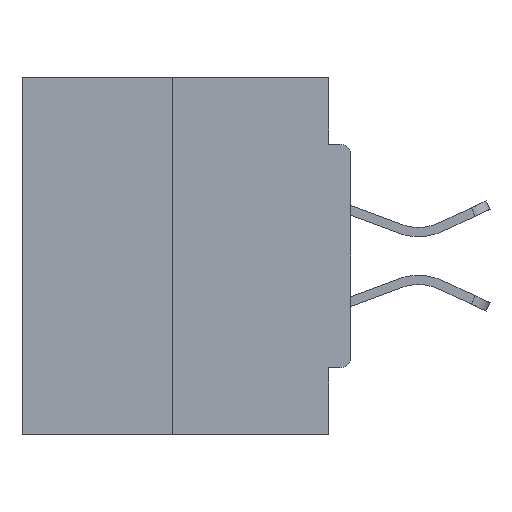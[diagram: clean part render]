
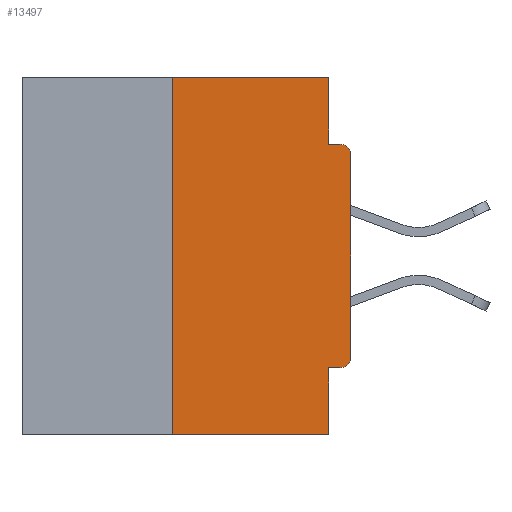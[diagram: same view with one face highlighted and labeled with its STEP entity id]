
A CAD part, left-side view. The second image highlights one B-rep face of the part: STEP entity #13497.
In plain terms, the highlighted planar face has unit normal (-1, 0, 0).
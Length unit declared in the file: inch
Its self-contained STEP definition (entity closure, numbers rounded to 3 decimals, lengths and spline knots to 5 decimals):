
#79 = EDGE_CURVE ( 'NONE', #23908, #3379, #25106, .T. ) ;
#124 = CIRCLE ( 'NONE', #31259, 0.015 ) ;
#161 = CARTESIAN_POINT ( 'NONE',  ( 0., 0.015, -0.1085 ) ) ;
#255 = CARTESIAN_POINT ( 'NONE',  ( 0., 0.031, -0.4065 ) ) ;
#318 = ORIENTED_EDGE ( 'NONE', *, *, #26460, .T. ) ;
#362 = ORIENTED_EDGE ( 'NONE', *, *, #3439, .T. ) ;
#2092 = DIRECTION ( 'NONE',  ( 0., 1., 0. ) ) ;
#2394 = LINE ( 'NONE', #14521, #20376 ) ;
#2426 = ORIENTED_EDGE ( 'NONE', *, *, #20431, .F. ) ;
#2506 = DIRECTION ( 'NONE',  ( 1., 0., 0. ) ) ;
#3024 = LINE ( 'NONE', #3363, #23427 ) ;
#3052 = DIRECTION ( 'NONE',  ( -1., 0., 0. ) ) ;
#3363 = CARTESIAN_POINT ( 'NONE',  ( 0., 0.46, 0. ) ) ;
#3379 = VERTEX_POINT ( 'NONE', #255 ) ;
#3439 = EDGE_CURVE ( 'NONE', #19172, #28922, #10156, .T. ) ;
#3564 = VECTOR ( 'NONE', #4030, 39.37008 ) ;
#4030 = DIRECTION ( 'NONE',  ( 0., -1., 0. ) ) ;
#4635 = EDGE_CURVE ( 'NONE', #23908, #19172, #124, .T. ) ;
#4663 = CARTESIAN_POINT ( 'NONE',  ( 0., 0.25, 0. ) ) ;
#4761 = VERTEX_POINT ( 'NONE', #15666 ) ;
#5387 = EDGE_CURVE ( 'NONE', #14861, #4761, #19274, .T. ) ;
#5404 = DIRECTION ( 'NONE',  ( 0., 0., 1. ) ) ;
#5481 = VECTOR ( 'NONE', #22290, 39.37008 ) ;
#6719 = DIRECTION ( 'NONE',  ( 0., -1., 0. ) ) ;
#7386 = AXIS2_PLACEMENT_3D ( 'NONE', #10082, #2506, #22948 ) ;
#8139 = EDGE_CURVE ( 'NONE', #4761, #22096, #31625, .T. ) ;
#8368 = ORIENTED_EDGE ( 'NONE', *, *, #8139, .F. ) ;
#8441 = CARTESIAN_POINT ( 'NONE',  ( 0., 0.031, -0.5 ) ) ;
#9300 = ORIENTED_EDGE ( 'NONE', *, *, #16008, .T. ) ;
#9609 = CIRCLE ( 'NONE', #29444, 0.015 ) ;
#9715 = CARTESIAN_POINT ( 'NONE',  ( 0., 0.015, -0.3915 ) ) ;
#9747 = ORIENTED_EDGE ( 'NONE', *, *, #79, .F. ) ;
#9770 = CARTESIAN_POINT ( 'NONE',  ( 0., 0., -0.4065 ) ) ;
#9828 = DIRECTION ( 'NONE',  ( -1., 0., 0. ) ) ;
#9996 = ORIENTED_EDGE ( 'NONE', *, *, #12390, .F. ) ;
#10082 = CARTESIAN_POINT ( 'NONE',  ( 0., 0.46, 0. ) ) ;
#10156 = LINE ( 'NONE', #28037, #21364 ) ;
#10636 = LINE ( 'NONE', #4663, #5481 ) ;
#10638 = VECTOR ( 'NONE', #21552, 39.37008 ) ;
#10709 = ORIENTED_EDGE ( 'NONE', *, *, #5387, .F. ) ;
#10846 = VECTOR ( 'NONE', #24326, 39.37008 ) ;
#11545 = CARTESIAN_POINT ( 'NONE',  ( 0., 0.031, 0. ) ) ;
#12390 = EDGE_CURVE ( 'NONE', #3379, #21579, #15863, .T. ) ;
#13497 = ADVANCED_FACE ( 'NONE', ( #29916 ), #25334, .F. ) ;
#14521 = CARTESIAN_POINT ( 'NONE',  ( 0., 0.46, -0.5 ) ) ;
#14584 = CARTESIAN_POINT ( 'NONE',  ( 0., 0.25, 0. ) ) ;
#14861 = VERTEX_POINT ( 'NONE', #29824 ) ;
#15666 = CARTESIAN_POINT ( 'NONE',  ( 0., 0.031, -0.0935 ) ) ;
#15863 = LINE ( 'NONE', #23798, #10638 ) ;
#16008 = EDGE_CURVE ( 'NONE', #28922, #22096, #9609, .T. ) ;
#16618 = CARTESIAN_POINT ( 'NONE',  ( 0., 0., -0.1085 ) ) ;
#16678 = VERTEX_POINT ( 'NONE', #24036 ) ;
#17970 = ORIENTED_EDGE ( 'NONE', *, *, #4635, .T. ) ;
#17991 = DIRECTION ( 'NONE',  ( 0., -1., 0. ) ) ;
#19172 = VERTEX_POINT ( 'NONE', #30401 ) ;
#19274 = LINE ( 'NONE', #11545, #10846 ) ;
#20376 = VECTOR ( 'NONE', #6719, 39.37008 ) ;
#20431 = EDGE_CURVE ( 'NONE', #16678, #30970, #10636, .T. ) ;
#20596 = DIRECTION ( 'NONE',  ( 0., 0., -1. ) ) ;
#21252 = EDGE_CURVE ( 'NONE', #30970, #14861, #3024, .T. ) ;
#21364 = VECTOR ( 'NONE', #5404, 39.37008 ) ;
#21552 = DIRECTION ( 'NONE',  ( 0., 0., -1. ) ) ;
#21571 = ORIENTED_EDGE ( 'NONE', *, *, #21252, .F. ) ;
#21579 = VERTEX_POINT ( 'NONE', #8441 ) ;
#21675 = EDGE_LOOP ( 'NONE', ( #21571, #2426, #318, #9996, #9747, #17970, #362, #9300, #8368, #10709 ) ) ;
#21836 = CARTESIAN_POINT ( 'NONE',  ( 0., 0.015, -0.4065 ) ) ;
#22010 = CARTESIAN_POINT ( 'NONE',  ( 0., 0.015, -0.0935 ) ) ;
#22096 = VERTEX_POINT ( 'NONE', #22010 ) ;
#22290 = DIRECTION ( 'NONE',  ( 0., 0., 1. ) ) ;
#22948 = DIRECTION ( 'NONE',  ( 0., 0., -1. ) ) ;
#23427 = VECTOR ( 'NONE', #17991, 39.37008 ) ;
#23798 = CARTESIAN_POINT ( 'NONE',  ( 0., 0.031, -0.5 ) ) ;
#23908 = VERTEX_POINT ( 'NONE', #21836 ) ;
#24036 = CARTESIAN_POINT ( 'NONE',  ( 0., 0.25, -0.5 ) ) ;
#24326 = DIRECTION ( 'NONE',  ( 0., 0., -1. ) ) ;
#25106 = LINE ( 'NONE', #9770, #30346 ) ;
#25334 = PLANE ( 'NONE',  #7386 ) ;
#26460 = EDGE_CURVE ( 'NONE', #16678, #21579, #2394, .T. ) ;
#27215 = CARTESIAN_POINT ( 'NONE',  ( 0., 0., -0.0935 ) ) ;
#27804 = DIRECTION ( 'NONE',  ( 0., 0., -1. ) ) ;
#28037 = CARTESIAN_POINT ( 'NONE',  ( 0., 0., 0. ) ) ;
#28922 = VERTEX_POINT ( 'NONE', #16618 ) ;
#29444 = AXIS2_PLACEMENT_3D ( 'NONE', #161, #3052, #20596 ) ;
#29824 = CARTESIAN_POINT ( 'NONE',  ( 0., 0.031, 0. ) ) ;
#29916 = FACE_OUTER_BOUND ( 'NONE', #21675, .T. ) ;
#30346 = VECTOR ( 'NONE', #2092, 39.37008 ) ;
#30401 = CARTESIAN_POINT ( 'NONE',  ( 0., 0., -0.3915 ) ) ;
#30970 = VERTEX_POINT ( 'NONE', #14584 ) ;
#31259 = AXIS2_PLACEMENT_3D ( 'NONE', #9715, #9828, #27804 ) ;
#31625 = LINE ( 'NONE', #27215, #3564 ) ;
